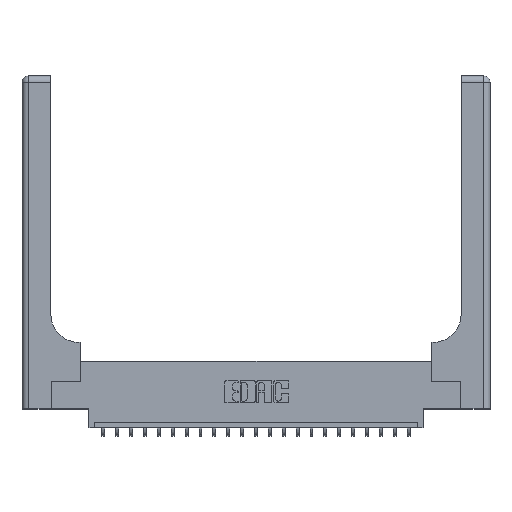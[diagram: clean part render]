
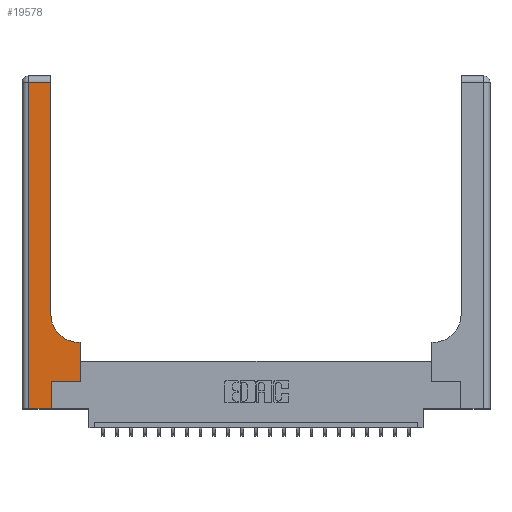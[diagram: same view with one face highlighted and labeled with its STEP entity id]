
A CAD part, top view. The second image highlights one B-rep face of the part: STEP entity #19578.
In plain terms, the highlighted planar face has unit normal (0, 0, 1).
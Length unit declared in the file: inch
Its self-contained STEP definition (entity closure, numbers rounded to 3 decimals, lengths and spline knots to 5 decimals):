
#444 = VECTOR ( 'NONE', #2197, 39.37008 ) ;
#768 = CARTESIAN_POINT ( 'NONE',  ( 0.26, 0.85, 0.37 ) ) ;
#803 = CARTESIAN_POINT ( 'NONE',  ( 0.06, 2.94, 0.37 ) ) ;
#1316 = VECTOR ( 'NONE', #15137, 39.37008 ) ;
#1341 = AXIS2_PLACEMENT_3D ( 'NONE', #1940, #7422, #15915 ) ;
#1543 = EDGE_CURVE ( 'NONE', #20647, #9947, #14773, .T. ) ;
#1940 = CARTESIAN_POINT ( 'NONE',  ( 0.51, 0.85, 0.37 ) ) ;
#2197 = DIRECTION ( 'NONE',  ( 0., 1., 0. ) ) ;
#2610 = CARTESIAN_POINT ( 'NONE',  ( 0.26, 2.94, 0.37 ) ) ;
#3795 = CARTESIAN_POINT ( 'NONE',  ( 0.265, 0., 0.37 ) ) ;
#3851 = LINE ( 'NONE', #13004, #17665 ) ;
#3931 = FACE_OUTER_BOUND ( 'NONE', #11937, .T. ) ;
#4542 = CARTESIAN_POINT ( 'NONE',  ( 0., 0., 0.37 ) ) ;
#5514 = CARTESIAN_POINT ( 'NONE',  ( 0.26, 0.6, 0.37 ) ) ;
#5681 = DIRECTION ( 'NONE',  ( 0., -1., 0. ) ) ;
#5999 = EDGE_CURVE ( 'NONE', #13657, #10767, #9820, .T. ) ;
#6059 = AXIS2_PLACEMENT_3D ( 'NONE', #7698, #10915, #14677 ) ;
#7203 = CARTESIAN_POINT ( 'NONE',  ( 0.06, 0., 0.37 ) ) ;
#7395 = DIRECTION ( 'NONE',  ( 0., 1., 0. ) ) ;
#7422 = DIRECTION ( 'NONE',  ( 0., 0., -1. ) ) ;
#7508 = LINE ( 'NONE', #21404, #17825 ) ;
#7698 = CARTESIAN_POINT ( 'NONE',  ( 0., 3., 0.37 ) ) ;
#7749 = EDGE_CURVE ( 'NONE', #10767, #21548, #12501, .T. ) ;
#7765 = EDGE_CURVE ( 'NONE', #9947, #22421, #10438, .T. ) ;
#8596 = EDGE_CURVE ( 'NONE', #18472, #19995, #3851, .T. ) ;
#9164 = ORIENTED_EDGE ( 'NONE', *, *, #21026, .T. ) ;
#9715 = ORIENTED_EDGE ( 'NONE', *, *, #5999, .T. ) ;
#9820 = LINE ( 'NONE', #4542, #12468 ) ;
#9947 = VERTEX_POINT ( 'NONE', #16922 ) ;
#10438 = LINE ( 'NONE', #5514, #16555 ) ;
#10767 = VERTEX_POINT ( 'NONE', #17517 ) ;
#10888 = DIRECTION ( 'NONE',  ( 0., 1., 0. ) ) ;
#10906 = ORIENTED_EDGE ( 'NONE', *, *, #1543, .T. ) ;
#10915 = DIRECTION ( 'NONE',  ( 0., 0., -1. ) ) ;
#11130 = PLANE ( 'NONE',  #6059 ) ;
#11183 = CIRCLE ( 'NONE', #1341, 0.25 ) ;
#11937 = EDGE_LOOP ( 'NONE', ( #18704, #9164, #12924, #9715, #17448, #21050, #10906, #17632, #16018 ) ) ;
#12121 = VERTEX_POINT ( 'NONE', #803 ) ;
#12358 = EDGE_CURVE ( 'NONE', #21548, #20647, #21099, .T. ) ;
#12468 = VECTOR ( 'NONE', #16819, 39.37008 ) ;
#12501 = LINE ( 'NONE', #3795, #15796 ) ;
#12924 = ORIENTED_EDGE ( 'NONE', *, *, #16787, .T. ) ;
#13004 = CARTESIAN_POINT ( 'NONE',  ( 0.26, 3., 0.37 ) ) ;
#13657 = VERTEX_POINT ( 'NONE', #7203 ) ;
#14677 = DIRECTION ( 'NONE',  ( -1., 0., 0. ) ) ;
#14773 = LINE ( 'NONE', #21800, #444 ) ;
#14914 = CARTESIAN_POINT ( 'NONE',  ( 0., 2.94, 0.37 ) ) ;
#15137 = DIRECTION ( 'NONE',  ( -1., 0., 0. ) ) ;
#15491 = CARTESIAN_POINT ( 'NONE',  ( 0.51, 0.6, 0.37 ) ) ;
#15574 = CARTESIAN_POINT ( 'NONE',  ( 0.265, 0.25, 0.37 ) ) ;
#15796 = VECTOR ( 'NONE', #10888, 39.37008 ) ;
#15799 = CARTESIAN_POINT ( 'NONE',  ( 0.265, 0.25, 0.37 ) ) ;
#15915 = DIRECTION ( 'NONE',  ( 1., 0., 0. ) ) ;
#16018 = ORIENTED_EDGE ( 'NONE', *, *, #21667, .T. ) ;
#16555 = VECTOR ( 'NONE', #17773, 39.37008 ) ;
#16638 = VECTOR ( 'NONE', #19253, 39.37008 ) ;
#16787 = EDGE_CURVE ( 'NONE', #12121, #13657, #7508, .T. ) ;
#16819 = DIRECTION ( 'NONE',  ( 1., 0., 0. ) ) ;
#16922 = CARTESIAN_POINT ( 'NONE',  ( 0.528, 0.6, 0.37 ) ) ;
#17448 = ORIENTED_EDGE ( 'NONE', *, *, #7749, .T. ) ;
#17517 = CARTESIAN_POINT ( 'NONE',  ( 0.265, 0., 0.37 ) ) ;
#17589 = CARTESIAN_POINT ( 'NONE',  ( 0.528, 0.25, 0.37 ) ) ;
#17632 = ORIENTED_EDGE ( 'NONE', *, *, #7765, .T. ) ;
#17665 = VECTOR ( 'NONE', #7395, 39.37008 ) ;
#17773 = DIRECTION ( 'NONE',  ( -1., 0., 0. ) ) ;
#17825 = VECTOR ( 'NONE', #5681, 39.37008 ) ;
#18472 = VERTEX_POINT ( 'NONE', #768 ) ;
#18704 = ORIENTED_EDGE ( 'NONE', *, *, #8596, .T. ) ;
#19253 = DIRECTION ( 'NONE',  ( 1., 0., 0. ) ) ;
#19578 = ADVANCED_FACE ( 'NONE', ( #3931 ), #11130, .F. ) ;
#19995 = VERTEX_POINT ( 'NONE', #2610 ) ;
#20444 = LINE ( 'NONE', #14914, #1316 ) ;
#20647 = VERTEX_POINT ( 'NONE', #17589 ) ;
#21026 = EDGE_CURVE ( 'NONE', #19995, #12121, #20444, .T. ) ;
#21050 = ORIENTED_EDGE ( 'NONE', *, *, #12358, .T. ) ;
#21099 = LINE ( 'NONE', #15799, #16638 ) ;
#21404 = CARTESIAN_POINT ( 'NONE',  ( 0.06, 3., 0.37 ) ) ;
#21548 = VERTEX_POINT ( 'NONE', #15574 ) ;
#21667 = EDGE_CURVE ( 'NONE', #22421, #18472, #11183, .T. ) ;
#21800 = CARTESIAN_POINT ( 'NONE',  ( 0.528, 0.25, 0.37 ) ) ;
#22421 = VERTEX_POINT ( 'NONE', #15491 ) ;
